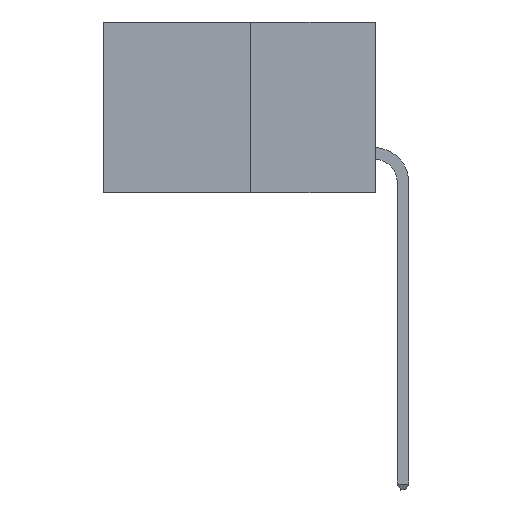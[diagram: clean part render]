
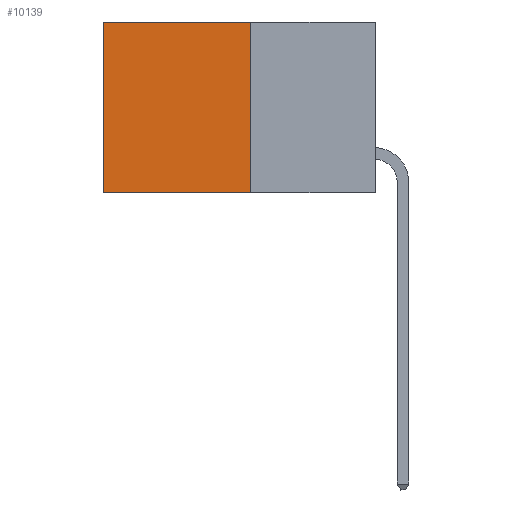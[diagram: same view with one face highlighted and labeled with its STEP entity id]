
A CAD part, left-side view. The second image highlights one B-rep face of the part: STEP entity #10139.
In plain terms, the highlighted planar face has unit normal (-1, 0, 0).
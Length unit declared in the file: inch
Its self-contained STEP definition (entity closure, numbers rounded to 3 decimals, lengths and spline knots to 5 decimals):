
#408 = CARTESIAN_POINT ( 'NONE',  ( 0.277, 0.27, 0. ) ) ;
#588 = VECTOR ( 'NONE', #19001, 39.37008 ) ;
#2747 = EDGE_LOOP ( 'NONE', ( #11261, #15724, #20177, #7873 ) ) ;
#3376 = PLANE ( 'NONE',  #9555 ) ;
#3520 = VECTOR ( 'NONE', #5048, 39.37008 ) ;
#4366 = VERTEX_POINT ( 'NONE', #14363 ) ;
#4861 = CARTESIAN_POINT ( 'NONE',  ( 0.277, 0.27, -0.37 ) ) ;
#5048 = DIRECTION ( 'NONE',  ( 0., 1., 0. ) ) ;
#5629 = LINE ( 'NONE', #17341, #588 ) ;
#7149 = LINE ( 'NONE', #21256, #19982 ) ;
#7873 = ORIENTED_EDGE ( 'NONE', *, *, #8991, .T. ) ;
#8482 = CARTESIAN_POINT ( 'NONE',  ( 0.277, 0.27, -0.37 ) ) ;
#8991 = EDGE_CURVE ( 'NONE', #18107, #15388, #17423, .T. ) ;
#9397 = DIRECTION ( 'NONE',  ( 0., 1., 0. ) ) ;
#9555 = AXIS2_PLACEMENT_3D ( 'NONE', #8482, #20199, #10137 ) ;
#10137 = DIRECTION ( 'NONE',  ( 0., 0., -1. ) ) ;
#10139 = ADVANCED_FACE ( 'NONE', ( #18687 ), #3376, .F. ) ;
#11261 = ORIENTED_EDGE ( 'NONE', *, *, #13891, .T. ) ;
#11400 = CARTESIAN_POINT ( 'NONE',  ( 0.277, 0.59, 0. ) ) ;
#12695 = VECTOR ( 'NONE', #9397, 39.37008 ) ;
#13633 = CARTESIAN_POINT ( 'NONE',  ( 0.277, 0.27, 0. ) ) ;
#13891 = EDGE_CURVE ( 'NONE', #15388, #4366, #5629, .T. ) ;
#14363 = CARTESIAN_POINT ( 'NONE',  ( 0.277, 0.59, -0.37 ) ) ;
#15312 = EDGE_CURVE ( 'NONE', #18107, #21694, #7149, .T. ) ;
#15388 = VERTEX_POINT ( 'NONE', #11400 ) ;
#15724 = ORIENTED_EDGE ( 'NONE', *, *, #20835, .F. ) ;
#16185 = DIRECTION ( 'NONE',  ( 0., 0., -1. ) ) ;
#17139 = LINE ( 'NONE', #17788, #12695 ) ;
#17341 = CARTESIAN_POINT ( 'NONE',  ( 0.277, 0.59, -0.37 ) ) ;
#17423 = LINE ( 'NONE', #13633, #3520 ) ;
#17788 = CARTESIAN_POINT ( 'NONE',  ( 0.277, 0.27, -0.37 ) ) ;
#18107 = VERTEX_POINT ( 'NONE', #408 ) ;
#18687 = FACE_OUTER_BOUND ( 'NONE', #2747, .T. ) ;
#19001 = DIRECTION ( 'NONE',  ( 0., 0., -1. ) ) ;
#19982 = VECTOR ( 'NONE', #16185, 39.37008 ) ;
#20177 = ORIENTED_EDGE ( 'NONE', *, *, #15312, .F. ) ;
#20199 = DIRECTION ( 'NONE',  ( 1., 0., 0. ) ) ;
#20835 = EDGE_CURVE ( 'NONE', #21694, #4366, #17139, .T. ) ;
#21256 = CARTESIAN_POINT ( 'NONE',  ( 0.277, 0.27, -0.37 ) ) ;
#21694 = VERTEX_POINT ( 'NONE', #4861 ) ;
